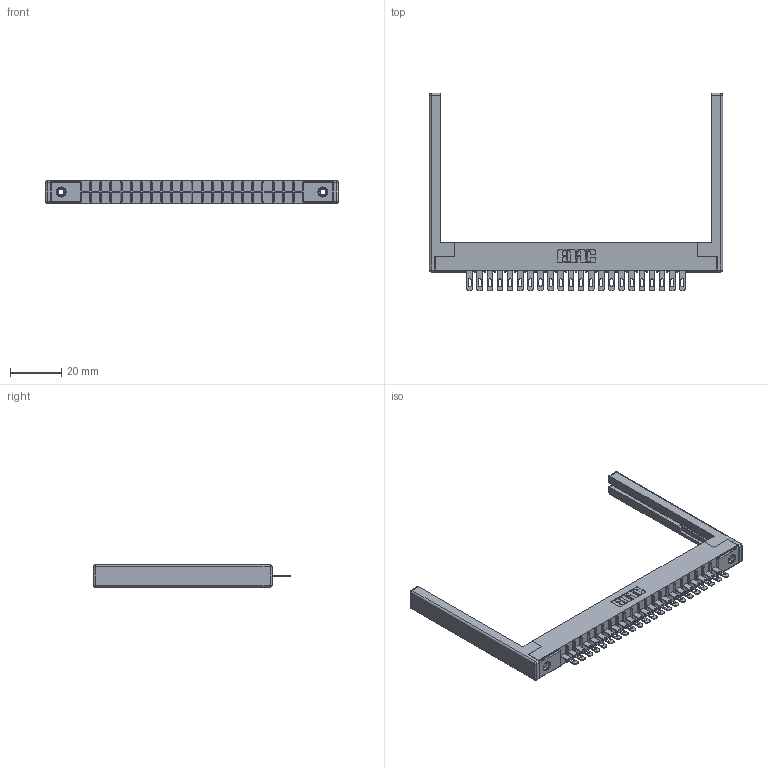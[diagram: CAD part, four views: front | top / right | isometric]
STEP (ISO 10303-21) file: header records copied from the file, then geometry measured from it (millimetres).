
FILE_DESCRIPTION (( 'STEP AP203' ), '1' );
FILE_NAME ('356-022-400-168.STEP', '2020-09-23T15:17:16', ( '' ), ( '' ), 'SwSTEP 2.0', 'SolidWorks 2020', '' );
FILE_SCHEMA (( 'CONFIG_CONTROL_DESIGN' ));
Length unit declared in the file: inch
Products named in the file (5): 306 Part_.156 Dia; 345-250-001_345-250-001-102; 307-220-068; 356-022-400-168; 306-290-001_100
Assembly tree (27 placements, depth 2):
  356-022-400-168
    306 Part_.156 Dia
    306-290-001_100  x22
    345-250-001_345-250-001-102  x2
    307-220-068  x2
Bounding box: 114.6 x 77.17 x 8.71 mm (x, y, z)
Volume: 12453.1 mm3; surface area: 16159.3 mm2
Topology: 27 solids, 27 shells, 1942 faces, 5436 edges, 3484 vertices
Faces by surface type: plane 1256, cylinder 574, sphere 96, cone 12, torus 4
Entity records: 26030 total; most frequent: CARTESIAN_POINT 4334, DIRECTION 4289, ORIENTED_EDGE 4286, EDGE_CURVE 2143, VECTOR 1659, LINE 1659, VERTEX_POINT 1360, AXIS2_PLACEMENT_3D 1315
